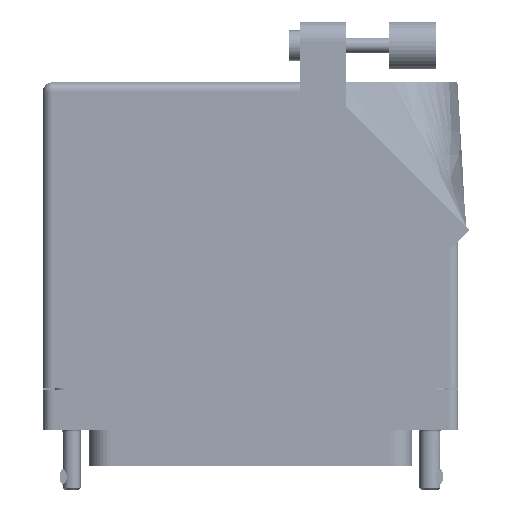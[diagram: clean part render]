
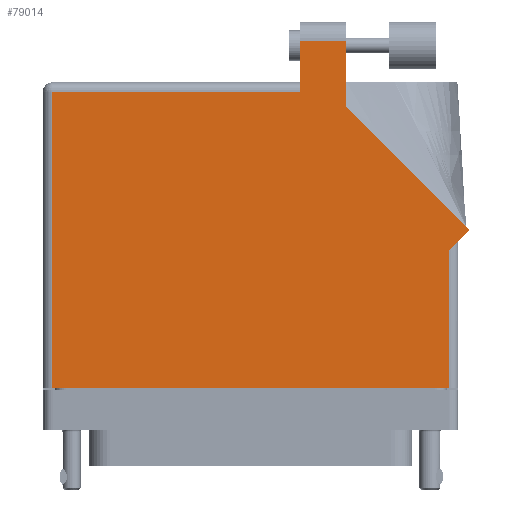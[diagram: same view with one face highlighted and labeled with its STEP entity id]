
A CAD part, front view. The second image highlights one B-rep face of the part: STEP entity #79014.
In plain terms, the highlighted face is planar.
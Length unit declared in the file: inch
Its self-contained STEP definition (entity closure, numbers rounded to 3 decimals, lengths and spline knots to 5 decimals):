
#2028 = VECTOR ( 'NONE', #53832, 39.37008 ) ;
#4661 = VERTEX_POINT ( 'NONE', #27450 ) ;
#8370 = DIRECTION ( 'NONE',  ( 0.707, 0.707, 0. ) ) ;
#9800 = FACE_OUTER_BOUND ( 'NONE', #23929, .T. ) ;
#13756 = ORIENTED_EDGE ( 'NONE', *, *, #94713, .T. ) ;
#14838 = VERTEX_POINT ( 'NONE', #58126 ) ;
#15078 = CARTESIAN_POINT ( 'NONE',  ( 0.3275, 2.205, 0.765 ) ) ;
#23929 = EDGE_LOOP ( 'NONE', ( #28086, #70668, #68328, #56889, #13756, #38546, #58987, #74390, #62046 ) ) ;
#24183 = VERTEX_POINT ( 'NONE', #83176 ) ;
#25855 = VECTOR ( 'NONE', #95901, 39.37008 ) ;
#27450 = CARTESIAN_POINT ( 'NONE',  ( 0.6345, 1.76442, 0.765 ) ) ;
#28086 = ORIENTED_EDGE ( 'NONE', *, *, #77522, .T. ) ;
#30774 = EDGE_CURVE ( 'NONE', #14838, #4661, #76666, .T. ) ;
#37524 = DIRECTION ( 'NONE',  ( -1., 0., 0. ) ) ;
#38546 = ORIENTED_EDGE ( 'NONE', *, *, #43638, .T. ) ;
#39563 = VERTEX_POINT ( 'NONE', #99580 ) ;
#41357 = DIRECTION ( 'NONE',  ( -1., 0., 0. ) ) ;
#43638 = EDGE_CURVE ( 'NONE', #89842, #68751, #86576, .T. ) ;
#48810 = VECTOR ( 'NONE', #95389, 39.37008 ) ;
#49811 = LINE ( 'NONE', #51151, #57224 ) ;
#50193 = VECTOR ( 'NONE', #8370, 39.37008 ) ;
#51151 = CARTESIAN_POINT ( 'NONE',  ( 0.3275, 1.93, 0.765 ) ) ;
#51212 = EDGE_CURVE ( 'NONE', #39563, #59388, #80163, .T. ) ;
#53832 = DIRECTION ( 'NONE',  ( 1., 0., 0. ) ) ;
#54515 = LINE ( 'NONE', #101513, #95581 ) ;
#56120 = DIRECTION ( 'NONE',  ( -0.707, 0.707, 0. ) ) ;
#56889 = ORIENTED_EDGE ( 'NONE', *, *, #91805, .T. ) ;
#57224 = VECTOR ( 'NONE', #97391, 39.37008 ) ;
#58126 = CARTESIAN_POINT ( 'NONE',  ( 1.44821, 0.95071, 0.765 ) ) ;
#58987 = ORIENTED_EDGE ( 'NONE', *, *, #92285, .T. ) ;
#59388 = VERTEX_POINT ( 'NONE', #15078 ) ;
#60574 = VECTOR ( 'NONE', #56120, 39.37008 ) ;
#62046 = ORIENTED_EDGE ( 'NONE', *, *, #30774, .T. ) ;
#62060 = DIRECTION ( 'NONE',  ( -1., 0., 0. ) ) ;
#62857 = CARTESIAN_POINT ( 'NONE',  ( 1.3775, 0.88, 0.765 ) ) ;
#63365 = CARTESIAN_POINT ( 'NONE',  ( 1.44821, 0.95071, 0.765 ) ) ;
#63546 = LINE ( 'NONE', #87431, #48810 ) ;
#63569 = PLANE ( 'NONE',  #70463 ) ;
#63937 = CARTESIAN_POINT ( 'NONE',  ( 1.3155, -0.1, 0.765 ) ) ;
#65638 = DIRECTION ( 'NONE',  ( 0., 0., -1. ) ) ;
#66480 = DIRECTION ( 'NONE',  ( 0., -1., 0. ) ) ;
#68328 = ORIENTED_EDGE ( 'NONE', *, *, #90111, .T. ) ;
#68751 = VERTEX_POINT ( 'NONE', #63937 ) ;
#69586 = VECTOR ( 'NONE', #66480, 39.37008 ) ;
#70463 = AXIS2_PLACEMENT_3D ( 'NONE', #71610, #65638, #41357 ) ;
#70668 = ORIENTED_EDGE ( 'NONE', *, *, #51212, .T. ) ;
#71610 = CARTESIAN_POINT ( 'NONE',  ( -1.3775, 1.93, 0.765 ) ) ;
#73339 = LINE ( 'NONE', #98150, #69586 ) ;
#74390 = ORIENTED_EDGE ( 'NONE', *, *, #87669, .T. ) ;
#74633 = CARTESIAN_POINT ( 'NONE',  ( 0.3275, 1.868, 0.765 ) ) ;
#76666 = LINE ( 'NONE', #63365, #60574 ) ;
#77522 = EDGE_CURVE ( 'NONE', #4661, #39563, #63546, .T. ) ;
#78783 = CARTESIAN_POINT ( 'NONE',  ( 0.3275, 2.205, 0.765 ) ) ;
#79014 = ADVANCED_FACE ( 'NONE', ( #9800 ), #63569, .F. ) ;
#80163 = LINE ( 'NONE', #78783, #93865 ) ;
#80245 = CARTESIAN_POINT ( 'NONE',  ( 1.3155, 0.88, 0.765 ) ) ;
#80285 = VERTEX_POINT ( 'NONE', #74633 ) ;
#82756 = CARTESIAN_POINT ( 'NONE',  ( 1.3155, 0.818, 0.765 ) ) ;
#83176 = CARTESIAN_POINT ( 'NONE',  ( -1.3155, 1.868, 0.765 ) ) ;
#85791 = CARTESIAN_POINT ( 'NONE',  ( -1.3775, -0.1, 0.765 ) ) ;
#86576 = LINE ( 'NONE', #85791, #2028 ) ;
#87431 = CARTESIAN_POINT ( 'NONE',  ( 0.6345, 1.76442, 0.765 ) ) ;
#87669 = EDGE_CURVE ( 'NONE', #90114, #14838, #93775, .T. ) ;
#89842 = VERTEX_POINT ( 'NONE', #96823 ) ;
#90111 = EDGE_CURVE ( 'NONE', #59388, #80285, #49811, .T. ) ;
#90114 = VERTEX_POINT ( 'NONE', #82756 ) ;
#91805 = EDGE_CURVE ( 'NONE', #80285, #24183, #54515, .T. ) ;
#92285 = EDGE_CURVE ( 'NONE', #68751, #90114, #97871, .T. ) ;
#93775 = LINE ( 'NONE', #62857, #50193 ) ;
#93865 = VECTOR ( 'NONE', #62060, 39.37008 ) ;
#94713 = EDGE_CURVE ( 'NONE', #24183, #89842, #73339, .T. ) ;
#95389 = DIRECTION ( 'NONE',  ( 0., 1., 0. ) ) ;
#95581 = VECTOR ( 'NONE', #37524, 39.37008 ) ;
#95901 = DIRECTION ( 'NONE',  ( 0., 1., 0. ) ) ;
#96823 = CARTESIAN_POINT ( 'NONE',  ( -1.3155, -0.1, 0.765 ) ) ;
#97391 = DIRECTION ( 'NONE',  ( 0., -1., 0. ) ) ;
#97871 = LINE ( 'NONE', #80245, #25855 ) ;
#98150 = CARTESIAN_POINT ( 'NONE',  ( -1.3155, -0.1, 0.765 ) ) ;
#99580 = CARTESIAN_POINT ( 'NONE',  ( 0.6345, 2.205, 0.765 ) ) ;
#101513 = CARTESIAN_POINT ( 'NONE',  ( -1.3775, 1.868, 0.765 ) ) ;
